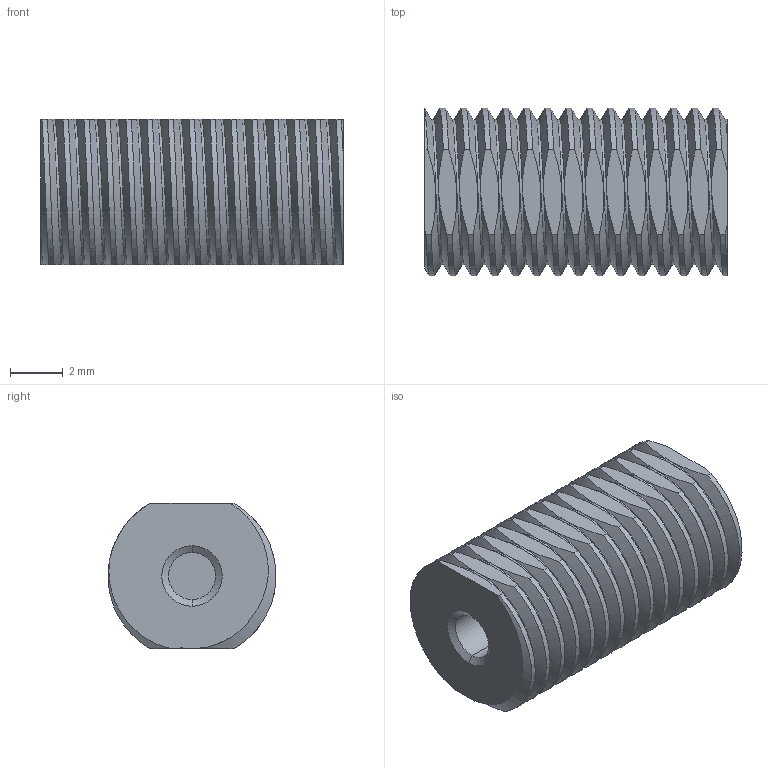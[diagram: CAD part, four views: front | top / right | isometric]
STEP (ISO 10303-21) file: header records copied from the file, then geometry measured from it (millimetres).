
FILE_DESCRIPTION (( 'STEP AP203' ), '1' );
FILE_NAME ('AF-WF-GS-PRT-004-STEP.STEP', '2020-07-21T18:59:12', ( '' ), ( '' ), 'SwSTEP 2.0', 'SolidWorks 2018', '' );
FILE_SCHEMA (( 'CONFIG_CONTROL_DESIGN' ));
Length unit declared in the file: inch
Products named in the file (1): AF-WF-GS-PRT-004-STEP
Bounding box: 11.43 x 6.34 x 5.49 mm (x, y, z)
Volume: 276 mm3; surface area: 447.6 mm2
Topology: 1 solids, 1 shells, 107 faces, 278 edges, 175 vertices
Faces by surface type: plane 37, cylinder 35, bspline 33, cone 2
Entity records: 20760 total; most frequent: CARTESIAN_POINT 18662, ORIENTED_EDGE 556, EDGE_CURVE 278, DIRECTION 254, VERTEX_POINT 175, EDGE_LOOP 109, ADVANCED_FACE 107, FACE_OUTER_BOUND 107
